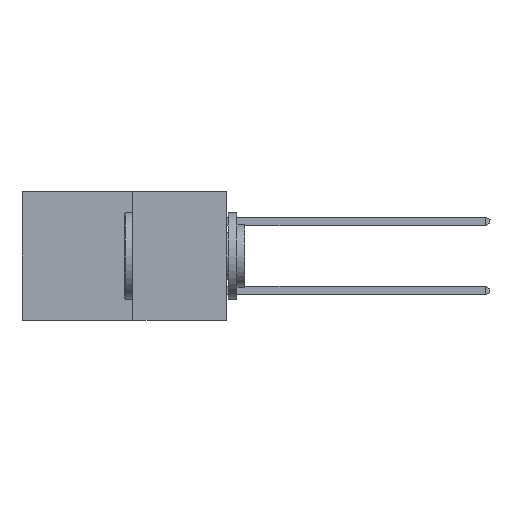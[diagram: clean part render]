
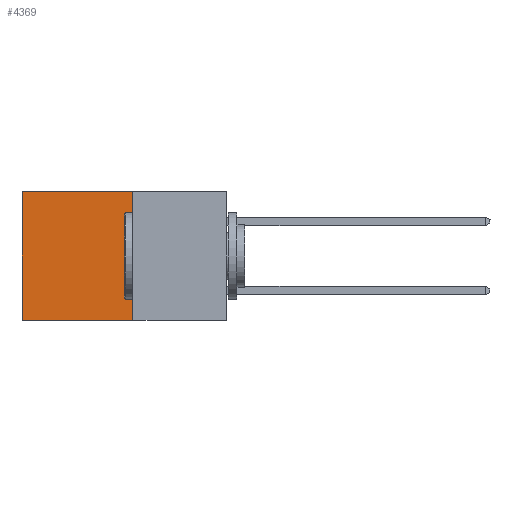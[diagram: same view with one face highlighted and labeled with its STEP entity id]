
A CAD part, left-side view. The second image highlights one B-rep face of the part: STEP entity #4369.
In plain terms, the highlighted planar face has unit normal (-1, 0, 0).
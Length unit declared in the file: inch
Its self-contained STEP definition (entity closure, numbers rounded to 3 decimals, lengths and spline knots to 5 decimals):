
#56 = LINE ( 'NONE', #5483, #7506 ) ;
#557 = EDGE_LOOP ( 'NONE', ( #8134, #733, #4619, #6510 ) ) ;
#733 = ORIENTED_EDGE ( 'NONE', *, *, #6487, .F. ) ;
#916 = VECTOR ( 'NONE', #6394, 39.37008 ) ;
#1191 = CARTESIAN_POINT ( 'NONE',  ( 0.277, 0.59, -0.37 ) ) ;
#2513 = DIRECTION ( 'NONE',  ( 0., 0., -1. ) ) ;
#2628 = DIRECTION ( 'NONE',  ( 1., 0., 0. ) ) ;
#2993 = PLANE ( 'NONE',  #4623 ) ;
#3133 = CARTESIAN_POINT ( 'NONE',  ( 0.277, 0.59, -0.37 ) ) ;
#3301 = FACE_OUTER_BOUND ( 'NONE', #557, .T. ) ;
#3349 = LINE ( 'NONE', #1191, #8713 ) ;
#3829 = LINE ( 'NONE', #6998, #7534 ) ;
#4042 = VERTEX_POINT ( 'NONE', #8873 ) ;
#4077 = DIRECTION ( 'NONE',  ( 0., 0., -1. ) ) ;
#4136 = DIRECTION ( 'NONE',  ( 0., 0., -1. ) ) ;
#4369 = ADVANCED_FACE ( 'NONE', ( #3301 ), #2993, .F. ) ;
#4410 = CARTESIAN_POINT ( 'NONE',  ( 0.277, 0.27, -0.37 ) ) ;
#4533 = VERTEX_POINT ( 'NONE', #7629 ) ;
#4619 = ORIENTED_EDGE ( 'NONE', *, *, #8553, .F. ) ;
#4623 = AXIS2_PLACEMENT_3D ( 'NONE', #4410, #2628, #2513 ) ;
#5483 = CARTESIAN_POINT ( 'NONE',  ( 0.277, 0.27, -0.37 ) ) ;
#6193 = CARTESIAN_POINT ( 'NONE',  ( 0.277, 0.27, -0.37 ) ) ;
#6389 = EDGE_CURVE ( 'NONE', #8026, #4533, #3829, .T. ) ;
#6394 = DIRECTION ( 'NONE',  ( 0., 1., 0. ) ) ;
#6487 = EDGE_CURVE ( 'NONE', #4042, #8994, #6676, .T. ) ;
#6510 = ORIENTED_EDGE ( 'NONE', *, *, #6389, .T. ) ;
#6676 = LINE ( 'NONE', #6193, #916 ) ;
#6998 = CARTESIAN_POINT ( 'NONE',  ( 0.277, 0.27, 0. ) ) ;
#7108 = DIRECTION ( 'NONE',  ( 0., 1., 0. ) ) ;
#7147 = CARTESIAN_POINT ( 'NONE',  ( 0.277, 0.27, 0. ) ) ;
#7506 = VECTOR ( 'NONE', #4077, 39.37008 ) ;
#7534 = VECTOR ( 'NONE', #7108, 39.37008 ) ;
#7629 = CARTESIAN_POINT ( 'NONE',  ( 0.277, 0.59, 0. ) ) ;
#8026 = VERTEX_POINT ( 'NONE', #7147 ) ;
#8134 = ORIENTED_EDGE ( 'NONE', *, *, #8612, .T. ) ;
#8553 = EDGE_CURVE ( 'NONE', #8026, #4042, #56, .T. ) ;
#8612 = EDGE_CURVE ( 'NONE', #4533, #8994, #3349, .T. ) ;
#8713 = VECTOR ( 'NONE', #4136, 39.37008 ) ;
#8873 = CARTESIAN_POINT ( 'NONE',  ( 0.277, 0.27, -0.37 ) ) ;
#8994 = VERTEX_POINT ( 'NONE', #3133 ) ;
